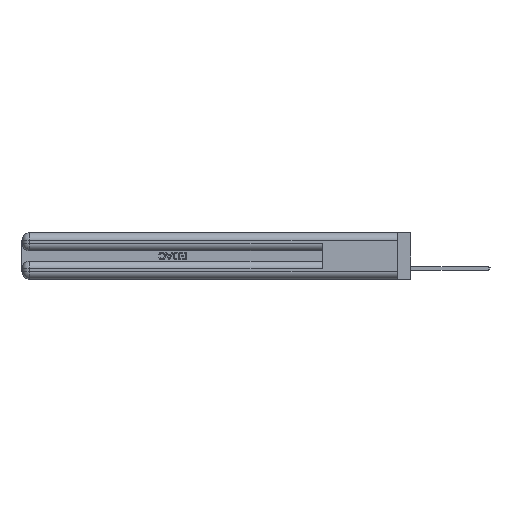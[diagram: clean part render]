
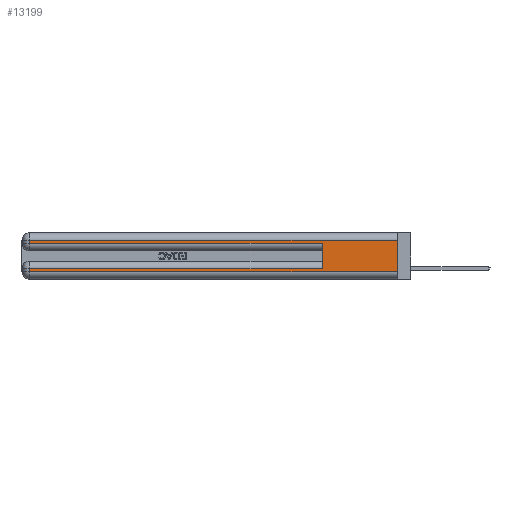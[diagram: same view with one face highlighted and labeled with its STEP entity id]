
A CAD part, left-side view. The second image highlights one B-rep face of the part: STEP entity #13199.
In plain terms, the highlighted planar face has unit normal (-1, 0, 0).
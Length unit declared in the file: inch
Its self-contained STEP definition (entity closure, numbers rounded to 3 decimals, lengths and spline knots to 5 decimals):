
#512 = FACE_OUTER_BOUND ( 'NONE', #44857, .T. ) ;
#826 = DIRECTION ( 'NONE',  ( 0., -1., 0. ) ) ;
#2605 = ORIENTED_EDGE ( 'NONE', *, *, #51037, .F. ) ;
#4131 = CARTESIAN_POINT ( 'NONE',  ( 0., 0., 0.06 ) ) ;
#4229 = ORIENTED_EDGE ( 'NONE', *, *, #41451, .T. ) ;
#4954 = LINE ( 'NONE', #11594, #52502 ) ;
#5989 = DIRECTION ( 'NONE',  ( 1., 0., 0. ) ) ;
#6965 = CARTESIAN_POINT ( 'NONE',  ( 0., 0., 0.37 ) ) ;
#7419 = VERTEX_POINT ( 'NONE', #31405 ) ;
#7966 = LINE ( 'NONE', #14758, #22658 ) ;
#8405 = LINE ( 'NONE', #53709, #27143 ) ;
#8638 = AXIS2_PLACEMENT_3D ( 'NONE', #12811, #5989, #31323 ) ;
#10985 = PLANE ( 'NONE',  #8638 ) ;
#11594 = CARTESIAN_POINT ( 'NONE',  ( 0., 0., 0.06 ) ) ;
#12811 = CARTESIAN_POINT ( 'NONE',  ( 0., 0., 0.37 ) ) ;
#13021 = CARTESIAN_POINT ( 'NONE',  ( 0., 0., 0.31 ) ) ;
#13139 = LINE ( 'NONE', #24814, #29332 ) ;
#13199 = ADVANCED_FACE ( 'NONE', ( #512 ), #10985, .F. ) ;
#13495 = LINE ( 'NONE', #13021, #51739 ) ;
#13633 = ORIENTED_EDGE ( 'NONE', *, *, #33527, .T. ) ;
#13806 = ORIENTED_EDGE ( 'NONE', *, *, #40038, .T. ) ;
#14362 = VERTEX_POINT ( 'NONE', #24101 ) ;
#14758 = CARTESIAN_POINT ( 'NONE',  ( 0., 2.94, 0.37 ) ) ;
#15809 = VERTEX_POINT ( 'NONE', #21930 ) ;
#16357 = EDGE_CURVE ( 'NONE', #15809, #19091, #4954, .T. ) ;
#19091 = VERTEX_POINT ( 'NONE', #4131 ) ;
#19116 = CARTESIAN_POINT ( 'NONE',  ( 0., 0.6, 0.145 ) ) ;
#21778 = LINE ( 'NONE', #6965, #54635 ) ;
#21930 = CARTESIAN_POINT ( 'NONE',  ( 0., 2.94, 0.06 ) ) ;
#22658 = VECTOR ( 'NONE', #26982, 39.37008 ) ;
#24101 = CARTESIAN_POINT ( 'NONE',  ( 0., 2.94, 0.31 ) ) ;
#24814 = CARTESIAN_POINT ( 'NONE',  ( 0., 2.94, 0.37 ) ) ;
#24822 = ORIENTED_EDGE ( 'NONE', *, *, #51119, .T. ) ;
#26769 = VERTEX_POINT ( 'NONE', #28151 ) ;
#26982 = DIRECTION ( 'NONE',  ( 0., 0., -1. ) ) ;
#27143 = VECTOR ( 'NONE', #27706, 39.37008 ) ;
#27706 = DIRECTION ( 'NONE',  ( 0., 1., 0. ) ) ;
#27920 = ORIENTED_EDGE ( 'NONE', *, *, #46642, .T. ) ;
#28134 = LINE ( 'NONE', #47377, #49532 ) ;
#28151 = CARTESIAN_POINT ( 'NONE',  ( 0., 0.6, 0.085 ) ) ;
#28297 = EDGE_CURVE ( 'NONE', #47597, #19091, #21778, .T. ) ;
#29332 = VECTOR ( 'NONE', #49655, 39.37008 ) ;
#30288 = DIRECTION ( 'NONE',  ( 0., 1., 0. ) ) ;
#31323 = DIRECTION ( 'NONE',  ( 0., 0., -1. ) ) ;
#31405 = CARTESIAN_POINT ( 'NONE',  ( 0., 2.94, 0.285 ) ) ;
#31496 = DIRECTION ( 'NONE',  ( 0., 0., 1. ) ) ;
#32114 = CARTESIAN_POINT ( 'NONE',  ( 0., 2.94, 0.085 ) ) ;
#33527 = EDGE_CURVE ( 'NONE', #14362, #7419, #13139, .T. ) ;
#33707 = ORIENTED_EDGE ( 'NONE', *, *, #16357, .T. ) ;
#37651 = DIRECTION ( 'NONE',  ( 0., -1., 0. ) ) ;
#40033 = ORIENTED_EDGE ( 'NONE', *, *, #28297, .F. ) ;
#40038 = EDGE_CURVE ( 'NONE', #47597, #14362, #13495, .T. ) ;
#41251 = DIRECTION ( 'NONE',  ( 0., 0., -1. ) ) ;
#41451 = EDGE_CURVE ( 'NONE', #7419, #41619, #28134, .T. ) ;
#41619 = VERTEX_POINT ( 'NONE', #52729 ) ;
#42362 = VERTEX_POINT ( 'NONE', #32114 ) ;
#44857 = EDGE_LOOP ( 'NONE', ( #40033, #13806, #13633, #4229, #2605, #27920, #24822, #33707 ) ) ;
#46642 = EDGE_CURVE ( 'NONE', #26769, #42362, #8405, .T. ) ;
#47377 = CARTESIAN_POINT ( 'NONE',  ( 0., 0., 0.285 ) ) ;
#47597 = VERTEX_POINT ( 'NONE', #48165 ) ;
#48165 = CARTESIAN_POINT ( 'NONE',  ( 0., 0., 0.31 ) ) ;
#49465 = LINE ( 'NONE', #19116, #54184 ) ;
#49532 = VECTOR ( 'NONE', #826, 39.37008 ) ;
#49655 = DIRECTION ( 'NONE',  ( 0., 0., -1. ) ) ;
#51037 = EDGE_CURVE ( 'NONE', #26769, #41619, #49465, .T. ) ;
#51119 = EDGE_CURVE ( 'NONE', #42362, #15809, #7966, .T. ) ;
#51739 = VECTOR ( 'NONE', #30288, 39.37008 ) ;
#52502 = VECTOR ( 'NONE', #37651, 39.37008 ) ;
#52729 = CARTESIAN_POINT ( 'NONE',  ( 0., 0.6, 0.285 ) ) ;
#53709 = CARTESIAN_POINT ( 'NONE',  ( 0., 0., 0.085 ) ) ;
#54184 = VECTOR ( 'NONE', #31496, 39.37008 ) ;
#54635 = VECTOR ( 'NONE', #41251, 39.37008 ) ;
